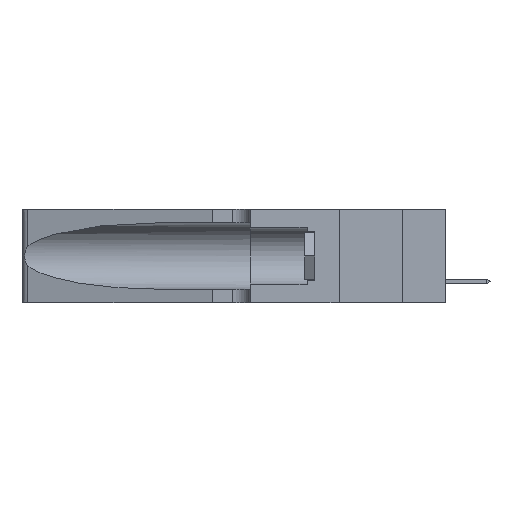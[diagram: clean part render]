
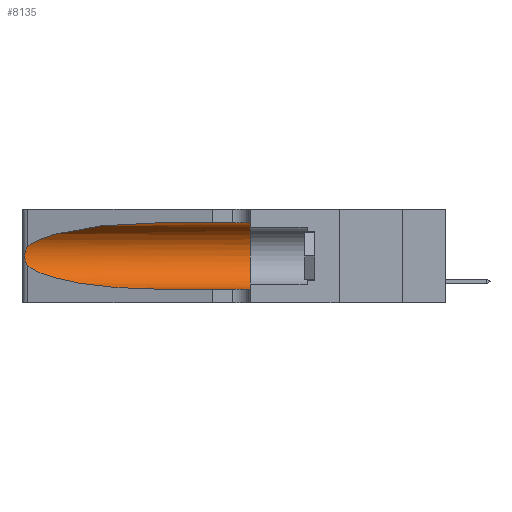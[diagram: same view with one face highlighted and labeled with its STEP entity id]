
A CAD part, left-side view. The second image highlights one B-rep face of the part: STEP entity #8135.
In plain terms, the highlighted cylindrical face has radius 3.308 mm (diameter 6.617 mm), a partial arc.
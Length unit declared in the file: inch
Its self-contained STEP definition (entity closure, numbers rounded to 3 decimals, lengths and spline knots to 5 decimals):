
#1332 = ORIENTED_EDGE ( 'NONE', *, *, #15834, .T. ) ;
#2090 = CARTESIAN_POINT ( 'NONE',  ( 0.2373, 1.15595, 0.08982 ) ) ;
#2817 = DIRECTION ( 'NONE',  ( 0., 0., -1. ) ) ;
#3190 = VERTEX_POINT ( 'NONE', #37066 ) ;
#5694 = VECTOR ( 'NONE', #39920, 39.37008 ) ;
#6453 = CARTESIAN_POINT ( 'NONE',  ( 0.18966, 0.96281, 0.31525 ) ) ;
#7377 = CYLINDRICAL_SURFACE ( 'NONE', #17197, 0.13025 ) ;
#7518 = CARTESIAN_POINT ( 'NONE',  ( 0.1305, 1.61858, 0.05475 ) ) ;
#8135 = ADVANCED_FACE ( 'NONE', ( #39688 ), #7377, .F. ) ;
#9217 = CARTESIAN_POINT ( 'NONE',  ( 0.25639, 1.23186, 0.15144 ) ) ;
#9488 = ORIENTED_EDGE ( 'NONE', *, *, #44718, .T. ) ;
#10483 = CARTESIAN_POINT ( 'NONE',  ( 0.25487, 1.22718, 0.22369 ) ) ;
#11091 = CARTESIAN_POINT ( 'NONE',  ( 0.1305, 1.61858, 0.185 ) ) ;
#11834 = CARTESIAN_POINT ( 'NONE',  ( 0.1305, 0.35, 0.05475 ) ) ;
#13100 = CARTESIAN_POINT ( 'NONE',  ( 0.26017, 1.23833, 0.17102 ) ) ;
#13438 = CARTESIAN_POINT ( 'NONE',  ( 0.25789, 1.23486, 0.15765 ) ) ;
#14485 = LINE ( 'NONE', #7518, #5694 ) ;
#15834 = EDGE_CURVE ( 'NONE', #40338, #3190, #37265, .T. ) ;
#16041 = CARTESIAN_POINT ( 'NONE',  ( 0.25487, 1.22718, 0.22369 ) ) ;
#16135 =( BOUNDED_CURVE ( )  B_SPLINE_CURVE ( 3, ( #50642, #2090, #46718, #26670 ),
 .UNSPECIFIED., .F., .F. ) 
 B_SPLINE_CURVE_WITH_KNOTS ( ( 4, 4 ),
 ( 3.44316, 4.71239 ),
 .UNSPECIFIED. ) 
 CURVE ( )  GEOMETRIC_REPRESENTATION_ITEM ( )  RATIONAL_B_SPLINE_CURVE ( ( 1., 0.87, 0.87, 1. ) ) 
 REPRESENTATION_ITEM ( '' )  );
#17197 = AXIS2_PLACEMENT_3D ( 'NONE', #11091, #43170, #2817 ) ;
#19066 = LINE ( 'NONE', #47501, #43148 ) ;
#20730 = ORIENTED_EDGE ( 'NONE', *, *, #48106, .F. ) ;
#20995 = VERTEX_POINT ( 'NONE', #11834 ) ;
#21429 = CARTESIAN_POINT ( 'NONE',  ( 0.25555, 1.22993, 0.14849 ) ) ;
#22123 = EDGE_CURVE ( 'NONE', #52323, #20995, #14485, .T. ) ;
#24820 = EDGE_LOOP ( 'NONE', ( #52173, #1332, #9488, #40981, #36968, #20730 ) ) ;
#24994 = CARTESIAN_POINT ( 'NONE',  ( 0.25639, 1.23184, 0.21858 ) ) ;
#25546 =( BOUNDED_CURVE ( )  B_SPLINE_CURVE ( 3, ( #39187, #6453, #30467, #10483 ),
 .UNSPECIFIED., .F., .T. ) 
 B_SPLINE_CURVE_WITH_KNOTS ( ( 4, 4 ),
 ( 1.5708, 2.84003 ),
 .UNSPECIFIED. ) 
 CURVE ( )  GEOMETRIC_REPRESENTATION_ITEM ( )  RATIONAL_B_SPLINE_CURVE ( ( 1., 0.87, 0.87, 1. ) ) 
 REPRESENTATION_ITEM ( '' )  );
#26670 = CARTESIAN_POINT ( 'NONE',  ( 0.1305, 0.72297, 0.05475 ) ) ;
#29054 = CARTESIAN_POINT ( 'NONE',  ( 0.25787, 1.23484, 0.2124 ) ) ;
#29385 = CARTESIAN_POINT ( 'NONE',  ( 0.26075, 1.23896, 0.178 ) ) ;
#30467 = CARTESIAN_POINT ( 'NONE',  ( 0.2373, 1.15595, 0.28018 ) ) ;
#30525 = DIRECTION ( 'NONE',  ( 0., 0., 1. ) ) ;
#30975 = CARTESIAN_POINT ( 'NONE',  ( 0.1305, 0.35, 0.31525 ) ) ;
#34127 = EDGE_CURVE ( 'NONE', #52291, #40338, #25546, .T. ) ;
#34165 = CARTESIAN_POINT ( 'NONE',  ( 0.25856, 1.23593, 0.16098 ) ) ;
#34646 = CARTESIAN_POINT ( 'NONE',  ( 0.1305, 0.35, 0.185 ) ) ;
#36882 = CARTESIAN_POINT ( 'NONE',  ( 0.25555, 1.22994, 0.2215 ) ) ;
#36968 = ORIENTED_EDGE ( 'NONE', *, *, #46668, .F. ) ;
#37066 = CARTESIAN_POINT ( 'NONE',  ( 0.25487, 1.22718, 0.14631 ) ) ;
#37265 = B_SPLINE_CURVE_WITH_KNOTS ( 'NONE', 3,
 ( #49317, #36882, #24994, #29054, #49657, #37749, #41805, #29385, #13100, #34165, #13438, #9217, #21429, #49837 ),
 .UNSPECIFIED., .F., .F.,
 ( 4, 2, 2, 2, 2, 2, 4 ),
 ( 0., 0.00027, 0.00053, 0.00107, 0.0016, 0.00187, 0.00214 ),
 .UNSPECIFIED. ) ;
#37749 = CARTESIAN_POINT ( 'NONE',  ( 0.26018, 1.23835, 0.19895 ) ) ;
#39187 = CARTESIAN_POINT ( 'NONE',  ( 0.1305, 0.72297, 0.31525 ) ) ;
#39661 = DIRECTION ( 'NONE',  ( 0., -1., 0. ) ) ;
#39688 = FACE_OUTER_BOUND ( 'NONE', #24820, .T. ) ;
#39816 = CARTESIAN_POINT ( 'NONE',  ( 0.1305, 0.72297, 0.05475 ) ) ;
#39920 = DIRECTION ( 'NONE',  ( 0., -1., 0. ) ) ;
#40338 = VERTEX_POINT ( 'NONE', #16041 ) ;
#40981 = ORIENTED_EDGE ( 'NONE', *, *, #22123, .T. ) ;
#41805 = CARTESIAN_POINT ( 'NONE',  ( 0.26075, 1.23896, 0.19203 ) ) ;
#42630 = VERTEX_POINT ( 'NONE', #30975 ) ;
#43148 = VECTOR ( 'NONE', #39661, 39.37008 ) ;
#43170 = DIRECTION ( 'NONE',  ( 0., -1., 0. ) ) ;
#43182 = CARTESIAN_POINT ( 'NONE',  ( 0.1305, 0.72297, 0.31525 ) ) ;
#44718 = EDGE_CURVE ( 'NONE', #3190, #52323, #16135, .T. ) ;
#46668 = EDGE_CURVE ( 'NONE', #42630, #20995, #52277, .T. ) ;
#46718 = CARTESIAN_POINT ( 'NONE',  ( 0.18966, 0.96281, 0.05475 ) ) ;
#47501 = CARTESIAN_POINT ( 'NONE',  ( 0.1305, 1.61858, 0.31525 ) ) ;
#48106 = EDGE_CURVE ( 'NONE', #52291, #42630, #19066, .T. ) ;
#49317 = CARTESIAN_POINT ( 'NONE',  ( 0.25487, 1.22718, 0.22369 ) ) ;
#49657 = CARTESIAN_POINT ( 'NONE',  ( 0.25854, 1.2359, 0.20912 ) ) ;
#49837 = CARTESIAN_POINT ( 'NONE',  ( 0.25487, 1.22718, 0.14631 ) ) ;
#50290 = AXIS2_PLACEMENT_3D ( 'NONE', #34646, #50831, #30525 ) ;
#50642 = CARTESIAN_POINT ( 'NONE',  ( 0.25487, 1.22718, 0.14631 ) ) ;
#50831 = DIRECTION ( 'NONE',  ( 0., 1., 0. ) ) ;
#52173 = ORIENTED_EDGE ( 'NONE', *, *, #34127, .T. ) ;
#52277 = CIRCLE ( 'NONE', #50290, 0.13025 ) ;
#52291 = VERTEX_POINT ( 'NONE', #43182 ) ;
#52323 = VERTEX_POINT ( 'NONE', #39816 ) ;
